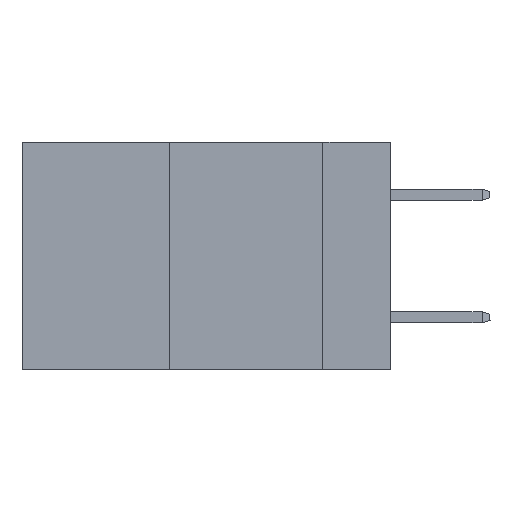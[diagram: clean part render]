
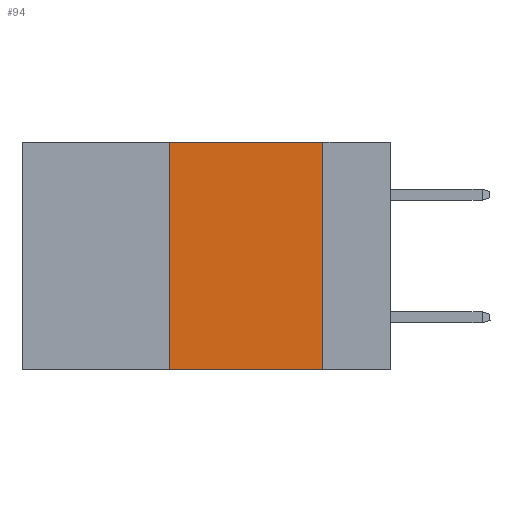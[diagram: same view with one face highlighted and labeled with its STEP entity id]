
A CAD part, left-side view. The second image highlights one B-rep face of the part: STEP entity #94.
In plain terms, the highlighted planar face has unit normal (-1, 0, 0).
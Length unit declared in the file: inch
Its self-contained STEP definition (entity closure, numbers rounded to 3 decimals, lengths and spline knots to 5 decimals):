
#94 = ADVANCED_FACE ( 'NONE', ( #13957 ), #3303, .F. ) ;
#549 = VECTOR ( 'NONE', #13685, 39.37008 ) ;
#2070 = VERTEX_POINT ( 'NONE', #3212 ) ;
#3169 = DIRECTION ( 'NONE',  ( 0., 0., -1. ) ) ;
#3212 = CARTESIAN_POINT ( 'NONE',  ( 0., 0.36, 0. ) ) ;
#3303 = PLANE ( 'NONE',  #18199 ) ;
#3373 = VECTOR ( 'NONE', #22830, 39.37008 ) ;
#3409 = DIRECTION ( 'NONE',  ( 1., 0., 0. ) ) ;
#3676 = CARTESIAN_POINT ( 'NONE',  ( 0., 0.36, -0.37 ) ) ;
#4530 = ORIENTED_EDGE ( 'NONE', *, *, #12770, .F. ) ;
#5384 = EDGE_LOOP ( 'NONE', ( #16403, #6807, #4530, #14555 ) ) ;
#6548 = CARTESIAN_POINT ( 'NONE',  ( 0., 0.36, 0. ) ) ;
#6807 = ORIENTED_EDGE ( 'NONE', *, *, #21064, .F. ) ;
#6982 = LINE ( 'NONE', #19641, #3373 ) ;
#8579 = EDGE_CURVE ( 'NONE', #10175, #19721, #19695, .T. ) ;
#9009 = CARTESIAN_POINT ( 'NONE',  ( 0., 0.11, 0. ) ) ;
#10175 = VERTEX_POINT ( 'NONE', #13479 ) ;
#12096 = DIRECTION ( 'NONE',  ( 0., 0., -1. ) ) ;
#12392 = LINE ( 'NONE', #12731, #22182 ) ;
#12731 = CARTESIAN_POINT ( 'NONE',  ( 0., 0.6, 0. ) ) ;
#12770 = EDGE_CURVE ( 'NONE', #14646, #2070, #22741, .T. ) ;
#13479 = CARTESIAN_POINT ( 'NONE',  ( 0., 0.11, 0. ) ) ;
#13685 = DIRECTION ( 'NONE',  ( 0., 0., 1. ) ) ;
#13957 = FACE_OUTER_BOUND ( 'NONE', #5384, .T. ) ;
#14253 = DIRECTION ( 'NONE',  ( 0., -1., 0. ) ) ;
#14555 = ORIENTED_EDGE ( 'NONE', *, *, #15754, .T. ) ;
#14646 = VERTEX_POINT ( 'NONE', #3676 ) ;
#14685 = VECTOR ( 'NONE', #3169, 39.37008 ) ;
#15754 = EDGE_CURVE ( 'NONE', #14646, #19721, #6982, .T. ) ;
#16403 = ORIENTED_EDGE ( 'NONE', *, *, #8579, .F. ) ;
#18199 = AXIS2_PLACEMENT_3D ( 'NONE', #23009, #3409, #12096 ) ;
#19534 = CARTESIAN_POINT ( 'NONE',  ( 0., 0.11, -0.37 ) ) ;
#19641 = CARTESIAN_POINT ( 'NONE',  ( 0., 0.6, -0.37 ) ) ;
#19695 = LINE ( 'NONE', #9009, #14685 ) ;
#19721 = VERTEX_POINT ( 'NONE', #19534 ) ;
#21064 = EDGE_CURVE ( 'NONE', #2070, #10175, #12392, .T. ) ;
#22182 = VECTOR ( 'NONE', #14253, 39.37008 ) ;
#22741 = LINE ( 'NONE', #6548, #549 ) ;
#22830 = DIRECTION ( 'NONE',  ( 0., -1., 0. ) ) ;
#23009 = CARTESIAN_POINT ( 'NONE',  ( 0., 0.6, 0. ) ) ;
